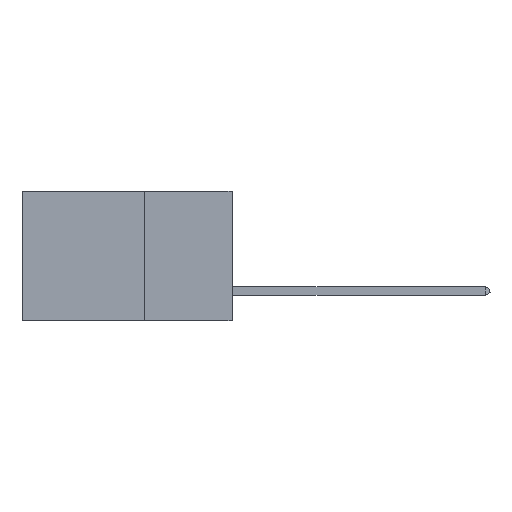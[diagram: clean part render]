
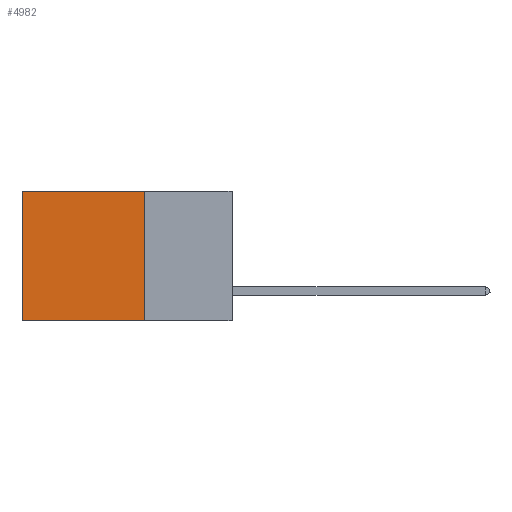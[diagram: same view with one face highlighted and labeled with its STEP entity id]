
A CAD part, left-side view. The second image highlights one B-rep face of the part: STEP entity #4982.
In plain terms, the highlighted planar face has unit normal (-1, 0, 0).
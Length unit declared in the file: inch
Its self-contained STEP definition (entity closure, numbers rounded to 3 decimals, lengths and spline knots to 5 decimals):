
#23 = VECTOR ( 'NONE', #337, 39.37008 ) ;
#337 = DIRECTION ( 'NONE',  ( 0., 0., -1. ) ) ;
#478 = CARTESIAN_POINT ( 'NONE',  ( 0.2875, 0.6, -0.37 ) ) ;
#924 = EDGE_CURVE ( 'NONE', #11668, #2598, #8567, .T. ) ;
#1316 = EDGE_CURVE ( 'NONE', #2598, #3903, #3377, .T. ) ;
#2598 = VERTEX_POINT ( 'NONE', #16621 ) ;
#3092 = VERTEX_POINT ( 'NONE', #16363 ) ;
#3377 = LINE ( 'NONE', #11035, #23 ) ;
#3481 = CARTESIAN_POINT ( 'NONE',  ( 0.2875, 0.25, 0. ) ) ;
#3510 = CARTESIAN_POINT ( 'NONE',  ( 0.2875, 0.25, 0. ) ) ;
#3716 = VECTOR ( 'NONE', #16901, 39.37008 ) ;
#3903 = VERTEX_POINT ( 'NONE', #478 ) ;
#3959 = AXIS2_PLACEMENT_3D ( 'NONE', #8298, #13538, #8188 ) ;
#4631 = VECTOR ( 'NONE', #7506, 39.37008 ) ;
#4982 = ADVANCED_FACE ( 'NONE', ( #13348 ), #17368, .F. ) ;
#5109 = ORIENTED_EDGE ( 'NONE', *, *, #8029, .F. ) ;
#6436 = VECTOR ( 'NONE', #7092, 39.37008 ) ;
#6724 = ORIENTED_EDGE ( 'NONE', *, *, #1316, .T. ) ;
#7092 = DIRECTION ( 'NONE',  ( 0., 1., 0. ) ) ;
#7321 = LINE ( 'NONE', #12551, #6436 ) ;
#7506 = DIRECTION ( 'NONE',  ( 0., 0., -1. ) ) ;
#8029 = EDGE_CURVE ( 'NONE', #3092, #3903, #7321, .T. ) ;
#8188 = DIRECTION ( 'NONE',  ( 0., 0., -1. ) ) ;
#8298 = CARTESIAN_POINT ( 'NONE',  ( 0.2875, 0.25, 0. ) ) ;
#8567 = LINE ( 'NONE', #3481, #3716 ) ;
#11035 = CARTESIAN_POINT ( 'NONE',  ( 0.2875, 0.6, 0. ) ) ;
#11573 = LINE ( 'NONE', #3510, #4631 ) ;
#11668 = VERTEX_POINT ( 'NONE', #14204 ) ;
#12215 = EDGE_CURVE ( 'NONE', #11668, #3092, #11573, .T. ) ;
#12551 = CARTESIAN_POINT ( 'NONE',  ( 0.2875, 0.25, -0.37 ) ) ;
#13348 = FACE_OUTER_BOUND ( 'NONE', #16471, .T. ) ;
#13538 = DIRECTION ( 'NONE',  ( 1., 0., 0. ) ) ;
#13764 = ORIENTED_EDGE ( 'NONE', *, *, #12215, .F. ) ;
#14204 = CARTESIAN_POINT ( 'NONE',  ( 0.2875, 0.25, 0. ) ) ;
#16069 = ORIENTED_EDGE ( 'NONE', *, *, #924, .T. ) ;
#16363 = CARTESIAN_POINT ( 'NONE',  ( 0.2875, 0.25, -0.37 ) ) ;
#16471 = EDGE_LOOP ( 'NONE', ( #6724, #5109, #13764, #16069 ) ) ;
#16621 = CARTESIAN_POINT ( 'NONE',  ( 0.2875, 0.6, 0. ) ) ;
#16901 = DIRECTION ( 'NONE',  ( 0., 1., 0. ) ) ;
#17368 = PLANE ( 'NONE',  #3959 ) ;
